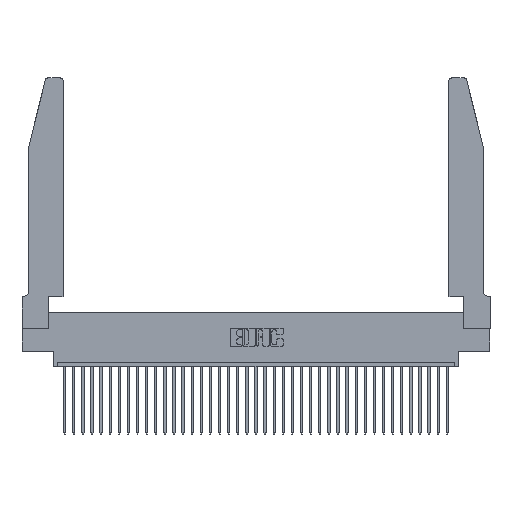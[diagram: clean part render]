
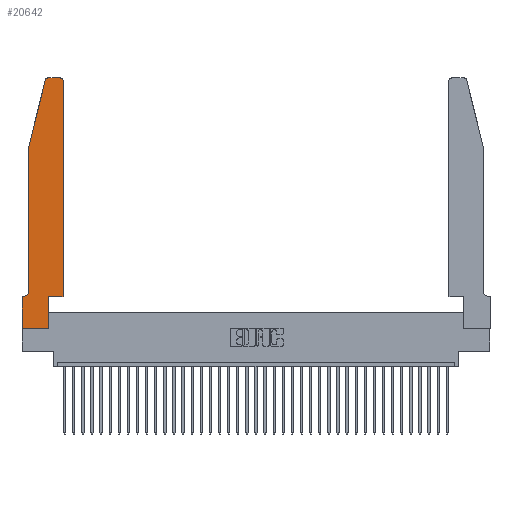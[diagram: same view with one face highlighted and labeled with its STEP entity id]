
A CAD part, top view. The second image highlights one B-rep face of the part: STEP entity #20642.
In plain terms, the highlighted planar face has unit normal (0, 0, 1).
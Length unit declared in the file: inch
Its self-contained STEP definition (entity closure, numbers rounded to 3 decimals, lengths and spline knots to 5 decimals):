
#715 = VERTEX_POINT ( 'NONE', #32248 ) ;
#907 = ORIENTED_EDGE ( 'NONE', *, *, #24014, .T. ) ;
#970 = FACE_OUTER_BOUND ( 'NONE', #23255, .T. ) ;
#978 = DIRECTION ( 'NONE',  ( 0., 1., 0. ) ) ;
#1816 = CARTESIAN_POINT ( 'NONE',  ( 0.0755, 0.35, 0.37 ) ) ;
#2016 = AXIS2_PLACEMENT_3D ( 'NONE', #2837, #19942, #22768 ) ;
#2189 = LINE ( 'NONE', #13621, #28086 ) ;
#2786 = LINE ( 'NONE', #11081, #13937 ) ;
#2837 = CARTESIAN_POINT ( 'NONE',  ( 0.4205, 2.72, 0.37 ) ) ;
#2854 = CIRCLE ( 'NONE', #2016, 0.03 ) ;
#3005 = ORIENTED_EDGE ( 'NONE', *, *, #26209, .T. ) ;
#4640 = LINE ( 'NONE', #5224, #5953 ) ;
#4712 = CARTESIAN_POINT ( 'NONE',  ( 0., 0.35, 0.37 ) ) ;
#4719 = LINE ( 'NONE', #29704, #34266 ) ;
#5224 = CARTESIAN_POINT ( 'NONE',  ( 0., 0., 0.37 ) ) ;
#5953 = VECTOR ( 'NONE', #10849, 39.37008 ) ;
#6800 = DIRECTION ( 'NONE',  ( 0., -1., 0. ) ) ;
#6959 = CARTESIAN_POINT ( 'NONE',  ( 0.0755, 2., 0.37 ) ) ;
#7524 = DIRECTION ( 'NONE',  ( -1., 0., 0. ) ) ;
#7945 = DIRECTION ( 'NONE',  ( 0., 0., -1. ) ) ;
#8021 = CARTESIAN_POINT ( 'NONE',  ( 0.2865, 0.35, 0.37 ) ) ;
#8297 = LINE ( 'NONE', #9822, #30254 ) ;
#9436 = DIRECTION ( 'NONE',  ( 0., -1., 0. ) ) ;
#9459 = CARTESIAN_POINT ( 'NONE',  ( 0.4505, 0.35, 0.37 ) ) ;
#9822 = CARTESIAN_POINT ( 'NONE',  ( 0.0755, 2., 0.37 ) ) ;
#10081 = DIRECTION ( 'NONE',  ( 1., 0., 0. ) ) ;
#10396 = DIRECTION ( 'NONE',  ( 0., 1., 0. ) ) ;
#10456 = CARTESIAN_POINT ( 'NONE',  ( 0.0055, 0.42, 0.37 ) ) ;
#10579 = DIRECTION ( 'NONE',  ( -1., 0., 0. ) ) ;
#10849 = DIRECTION ( 'NONE',  ( 1., 0., 0. ) ) ;
#11019 = VECTOR ( 'NONE', #7524, 39.37008 ) ;
#11034 = ORIENTED_EDGE ( 'NONE', *, *, #15257, .T. ) ;
#11081 = CARTESIAN_POINT ( 'NONE',  ( 0.0755, 2., 0.37 ) ) ;
#11578 = VECTOR ( 'NONE', #978, 39.37008 ) ;
#12177 = EDGE_CURVE ( 'NONE', #31509, #30836, #14257, .T. ) ;
#12261 = VECTOR ( 'NONE', #6800, 39.37008 ) ;
#12397 = CARTESIAN_POINT ( 'NONE',  ( 0.2865, 0., 0.37 ) ) ;
#13031 = CARTESIAN_POINT ( 'NONE',  ( 0.4205, 2.75, 0.37 ) ) ;
#13193 = VERTEX_POINT ( 'NONE', #13031 ) ;
#13621 = CARTESIAN_POINT ( 'NONE',  ( 0.4505, 0.35, 0.37 ) ) ;
#13937 = VECTOR ( 'NONE', #27726, 39.37008 ) ;
#14138 = EDGE_CURVE ( 'NONE', #715, #30816, #25758, .T. ) ;
#14257 = LINE ( 'NONE', #9459, #11578 ) ;
#15257 = EDGE_CURVE ( 'NONE', #30836, #13193, #2854, .T. ) ;
#15401 = ORIENTED_EDGE ( 'NONE', *, *, #30822, .T. ) ;
#16065 = ORIENTED_EDGE ( 'NONE', *, *, #17023, .T. ) ;
#16174 = VERTEX_POINT ( 'NONE', #37085 ) ;
#16411 = AXIS2_PLACEMENT_3D ( 'NONE', #21539, #35919, #10081 ) ;
#16561 = CARTESIAN_POINT ( 'NONE',  ( 0.4505, 2.72, 0.37 ) ) ;
#16805 = ORIENTED_EDGE ( 'NONE', *, *, #14138, .T. ) ;
#17023 = EDGE_CURVE ( 'NONE', #31532, #21920, #2786, .T. ) ;
#17637 = DIRECTION ( 'NONE',  ( 1., 0., 0. ) ) ;
#17657 = CARTESIAN_POINT ( 'NONE',  ( 0.2865, 0.35, 0.37 ) ) ;
#19942 = DIRECTION ( 'NONE',  ( 0., 0., 1. ) ) ;
#20346 = VERTEX_POINT ( 'NONE', #17657 ) ;
#20370 = ORIENTED_EDGE ( 'NONE', *, *, #28848, .T. ) ;
#20642 = ADVANCED_FACE ( 'NONE', ( #970 ), #21669, .T. ) ;
#21152 = CARTESIAN_POINT ( 'NONE',  ( 0., 0., 0.37 ) ) ;
#21539 = CARTESIAN_POINT ( 'NONE',  ( 0., 0.35, 0.37 ) ) ;
#21669 = PLANE ( 'NONE',  #16411 ) ;
#21920 = VERTEX_POINT ( 'NONE', #6959 ) ;
#22038 = DIRECTION ( 'NONE',  ( -1., 0., 0. ) ) ;
#22201 = ORIENTED_EDGE ( 'NONE', *, *, #27866, .T. ) ;
#22749 = CARTESIAN_POINT ( 'NONE',  ( 0.4505, 0.35, 0.37 ) ) ;
#22768 = DIRECTION ( 'NONE',  ( 1., 0., 0. ) ) ;
#22996 = VECTOR ( 'NONE', #10396, 39.37008 ) ;
#23210 = CARTESIAN_POINT ( 'NONE',  ( 0.284, 2.72, 0.37 ) ) ;
#23255 = EDGE_LOOP ( 'NONE', ( #3005, #23261, #16065, #907, #15401, #16805, #29075, #20370, #22201, #32884, #33002, #11034 ) ) ;
#23261 = ORIENTED_EDGE ( 'NONE', *, *, #29680, .T. ) ;
#24014 = EDGE_CURVE ( 'NONE', #21920, #30292, #8297, .T. ) ;
#24285 = EDGE_CURVE ( 'NONE', #30816, #28319, #33820, .T. ) ;
#25758 = LINE ( 'NONE', #1816, #11019 ) ;
#25835 = VERTEX_POINT ( 'NONE', #12397 ) ;
#26009 = CIRCLE ( 'NONE', #29271, 0.03 ) ;
#26209 = EDGE_CURVE ( 'NONE', #13193, #16174, #4719, .T. ) ;
#27726 = DIRECTION ( 'NONE',  ( -0.239, -0.971, 0. ) ) ;
#27866 = EDGE_CURVE ( 'NONE', #25835, #20346, #32006, .T. ) ;
#28086 = VECTOR ( 'NONE', #31029, 39.37008 ) ;
#28319 = VERTEX_POINT ( 'NONE', #28731 ) ;
#28731 = CARTESIAN_POINT ( 'NONE',  ( 0., 0., 0.37 ) ) ;
#28848 = EDGE_CURVE ( 'NONE', #28319, #25835, #4640, .T. ) ;
#29075 = ORIENTED_EDGE ( 'NONE', *, *, #24285, .T. ) ;
#29271 = AXIS2_PLACEMENT_3D ( 'NONE', #23210, #34830, #17637 ) ;
#29680 = EDGE_CURVE ( 'NONE', #16174, #31532, #26009, .T. ) ;
#29704 = CARTESIAN_POINT ( 'NONE',  ( 0.2605, 2.75, 0.37 ) ) ;
#30108 = CARTESIAN_POINT ( 'NONE',  ( 0.25487, 2.72718, 0.37 ) ) ;
#30254 = VECTOR ( 'NONE', #9436, 39.37008 ) ;
#30292 = VERTEX_POINT ( 'NONE', #34782 ) ;
#30816 = VERTEX_POINT ( 'NONE', #4712 ) ;
#30822 = EDGE_CURVE ( 'NONE', #30292, #715, #35730, .T. ) ;
#30836 = VERTEX_POINT ( 'NONE', #16561 ) ;
#31029 = DIRECTION ( 'NONE',  ( 1., 0., 0. ) ) ;
#31509 = VERTEX_POINT ( 'NONE', #22749 ) ;
#31532 = VERTEX_POINT ( 'NONE', #30108 ) ;
#32006 = LINE ( 'NONE', #8021, #22996 ) ;
#32198 = AXIS2_PLACEMENT_3D ( 'NONE', #10456, #7945, #10579 ) ;
#32248 = CARTESIAN_POINT ( 'NONE',  ( 0.0055, 0.35, 0.37 ) ) ;
#32884 = ORIENTED_EDGE ( 'NONE', *, *, #35659, .T. ) ;
#33002 = ORIENTED_EDGE ( 'NONE', *, *, #12177, .T. ) ;
#33820 = LINE ( 'NONE', #21152, #12261 ) ;
#34266 = VECTOR ( 'NONE', #22038, 39.37008 ) ;
#34782 = CARTESIAN_POINT ( 'NONE',  ( 0.0755, 0.42, 0.37 ) ) ;
#34830 = DIRECTION ( 'NONE',  ( 0., 0., 1. ) ) ;
#35659 = EDGE_CURVE ( 'NONE', #20346, #31509, #2189, .T. ) ;
#35730 = CIRCLE ( 'NONE', #32198, 0.07 ) ;
#35919 = DIRECTION ( 'NONE',  ( 0., 0., 1. ) ) ;
#37085 = CARTESIAN_POINT ( 'NONE',  ( 0.284, 2.75, 0.37 ) ) ;
